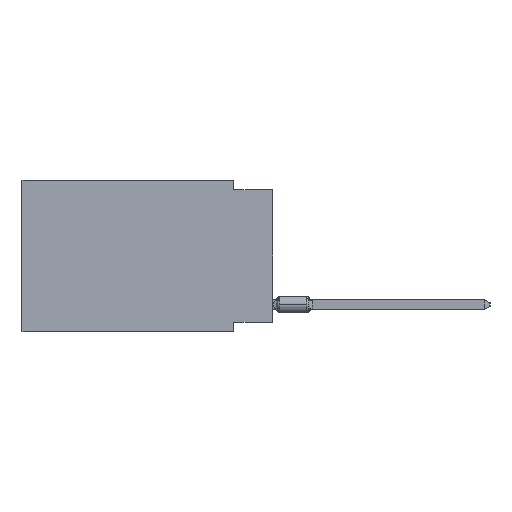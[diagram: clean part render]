
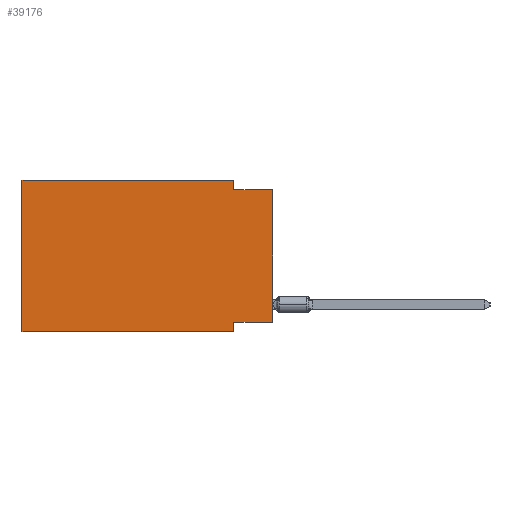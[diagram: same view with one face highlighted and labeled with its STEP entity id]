
A CAD part, left-side view. The second image highlights one B-rep face of the part: STEP entity #39176.
In plain terms, the highlighted planar face has unit normal (-1, 0, 0).
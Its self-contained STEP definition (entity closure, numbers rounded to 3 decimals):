
#298 = CARTESIAN_POINT ( 'NONE',  ( 0., 2.54, 0. ) ) ;
#627 = LINE ( 'NONE', #298, #36466 ) ;
#1379 = VERTEX_POINT ( 'NONE', #22237 ) ;
#2516 = EDGE_CURVE ( 'NONE', #60022, #29313, #40039, .T. ) ;
#4716 = LINE ( 'NONE', #9951, #61555 ) ;
#5630 = DIRECTION ( 'NONE',  ( 0., -1., 0. ) ) ;
#6143 = LINE ( 'NONE', #32355, #34541 ) ;
#6761 = EDGE_CURVE ( 'NONE', #48492, #54178, #4716, .T. ) ;
#7121 = VECTOR ( 'NONE', #31086, 1000. ) ;
#7714 = CARTESIAN_POINT ( 'NONE',  ( 0., 0., -0.635 ) ) ;
#7761 = ORIENTED_EDGE ( 'NONE', *, *, #36561, .F. ) ;
#9951 = CARTESIAN_POINT ( 'NONE',  ( 0., 16.383, 0. ) ) ;
#10099 = LINE ( 'NONE', #53730, #60946 ) ;
#11902 = EDGE_CURVE ( 'NONE', #54178, #60022, #627, .T. ) ;
#14365 = DIRECTION ( 'NONE',  ( 0., -1., 0. ) ) ;
#14678 = FACE_OUTER_BOUND ( 'NONE', #19019, .T. ) ;
#15806 = LINE ( 'NONE', #34834, #59876 ) ;
#19019 = EDGE_LOOP ( 'NONE', ( #28491, #60813, #43647, #20159, #7761, #31341, #59156, #30911 ) ) ;
#20159 = ORIENTED_EDGE ( 'NONE', *, *, #6761, .F. ) ;
#20914 = DIRECTION ( 'NONE',  ( 0., 0., -1. ) ) ;
#22214 = DIRECTION ( 'NONE',  ( 0., 1., 0. ) ) ;
#22237 = CARTESIAN_POINT ( 'NONE',  ( 0., 0., -9.271 ) ) ;
#23730 = DIRECTION ( 'NONE',  ( 0., -1., 0. ) ) ;
#23789 = DIRECTION ( 'NONE',  ( 0., 0., 1. ) ) ;
#24139 = VERTEX_POINT ( 'NONE', #29146 ) ;
#27663 = CARTESIAN_POINT ( 'NONE',  ( 0., 2.54, -0.635 ) ) ;
#28491 = ORIENTED_EDGE ( 'NONE', *, *, #30478, .T. ) ;
#29146 = CARTESIAN_POINT ( 'NONE',  ( 0., 2.54, -9.906 ) ) ;
#29313 = VERTEX_POINT ( 'NONE', #7714 ) ;
#29439 = PLANE ( 'NONE',  #61102 ) ;
#30478 = EDGE_CURVE ( 'NONE', #1379, #29313, #44451, .T. ) ;
#30911 = ORIENTED_EDGE ( 'NONE', *, *, #47551, .F. ) ;
#31086 = DIRECTION ( 'NONE',  ( 0., 0., -1. ) ) ;
#31341 = ORIENTED_EDGE ( 'NONE', *, *, #56887, .T. ) ;
#31570 = CARTESIAN_POINT ( 'NONE',  ( 0., 2.54, -9.271 ) ) ;
#32355 = CARTESIAN_POINT ( 'NONE',  ( 0., 0., -9.271 ) ) ;
#33898 = VECTOR ( 'NONE', #5630, 1000. ) ;
#34382 = CARTESIAN_POINT ( 'NONE',  ( 0., 2.54, -9.906 ) ) ;
#34541 = VECTOR ( 'NONE', #22214, 1000. ) ;
#34834 = CARTESIAN_POINT ( 'NONE',  ( 0., 16.383, 0. ) ) ;
#35323 = CARTESIAN_POINT ( 'NONE',  ( 0., 16.383, 0. ) ) ;
#36114 = CARTESIAN_POINT ( 'NONE',  ( 0., 0., -0.635 ) ) ;
#36466 = VECTOR ( 'NONE', #20914, 1000. ) ;
#36561 = EDGE_CURVE ( 'NONE', #63668, #48492, #15806, .T. ) ;
#39176 = ADVANCED_FACE ( 'NONE', ( #14678 ), #29439, .F. ) ;
#40039 = LINE ( 'NONE', #36114, #33898 ) ;
#40164 = VERTEX_POINT ( 'NONE', #31570 ) ;
#43647 = ORIENTED_EDGE ( 'NONE', *, *, #11902, .F. ) ;
#44451 = LINE ( 'NONE', #49997, #46008 ) ;
#46008 = VECTOR ( 'NONE', #23789, 1000. ) ;
#46511 = CARTESIAN_POINT ( 'NONE',  ( 0., 2.54, 0. ) ) ;
#47551 = EDGE_CURVE ( 'NONE', #1379, #40164, #6143, .T. ) ;
#48492 = VERTEX_POINT ( 'NONE', #63360 ) ;
#49442 = DIRECTION ( 'NONE',  ( 1., 0., 0. ) ) ;
#49997 = CARTESIAN_POINT ( 'NONE',  ( 0., 0., 0. ) ) ;
#50338 = EDGE_CURVE ( 'NONE', #40164, #24139, #59331, .T. ) ;
#53730 = CARTESIAN_POINT ( 'NONE',  ( 0., 16.383, -9.906 ) ) ;
#54178 = VERTEX_POINT ( 'NONE', #46511 ) ;
#54840 = DIRECTION ( 'NONE',  ( 0., 0., 1. ) ) ;
#56887 = EDGE_CURVE ( 'NONE', #63668, #24139, #10099, .T. ) ;
#59156 = ORIENTED_EDGE ( 'NONE', *, *, #50338, .F. ) ;
#59331 = LINE ( 'NONE', #34382, #7121 ) ;
#59876 = VECTOR ( 'NONE', #54840, 1000. ) ;
#60022 = VERTEX_POINT ( 'NONE', #27663 ) ;
#60048 = CARTESIAN_POINT ( 'NONE',  ( 0., 16.383, -9.906 ) ) ;
#60277 = DIRECTION ( 'NONE',  ( 0., 0., -1. ) ) ;
#60813 = ORIENTED_EDGE ( 'NONE', *, *, #2516, .F. ) ;
#60946 = VECTOR ( 'NONE', #14365, 1000. ) ;
#61102 = AXIS2_PLACEMENT_3D ( 'NONE', #35323, #49442, #60277 ) ;
#61555 = VECTOR ( 'NONE', #23730, 1000. ) ;
#63360 = CARTESIAN_POINT ( 'NONE',  ( 0., 16.383, 0. ) ) ;
#63668 = VERTEX_POINT ( 'NONE', #60048 ) ;
